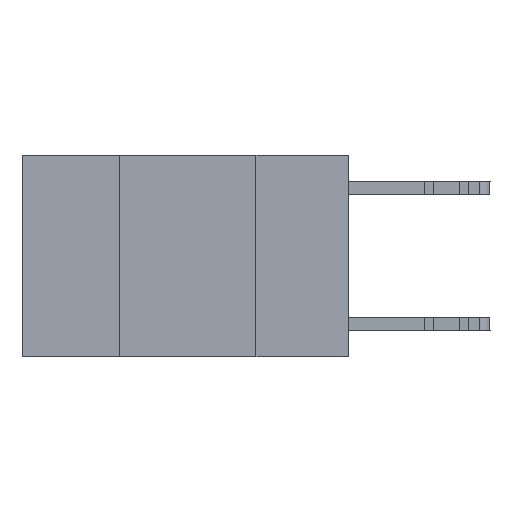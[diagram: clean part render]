
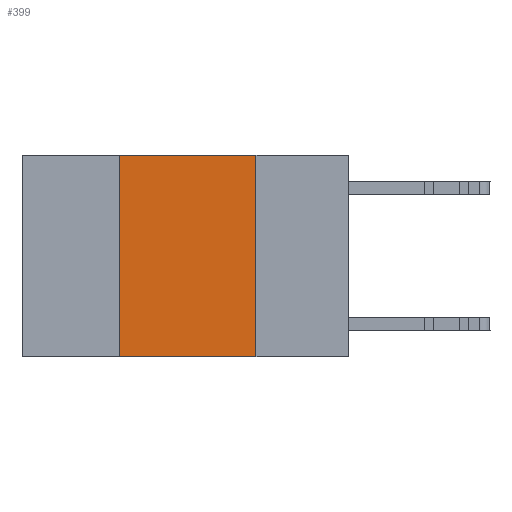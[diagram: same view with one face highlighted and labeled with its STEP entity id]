
A CAD part, left-side view. The second image highlights one B-rep face of the part: STEP entity #399.
In plain terms, the highlighted planar face has unit normal (-1, 0, 0).
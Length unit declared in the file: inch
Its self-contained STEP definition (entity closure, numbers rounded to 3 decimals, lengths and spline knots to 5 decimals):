
#399 = ADVANCED_FACE ( 'NONE', ( #556 ), #14731, .F. ) ;
#556 = FACE_OUTER_BOUND ( 'NONE', #13640, .T. ) ;
#1624 = VERTEX_POINT ( 'NONE', #8422 ) ;
#3134 = CARTESIAN_POINT ( 'NONE',  ( 0., 0.17, 0. ) ) ;
#4182 = DIRECTION ( 'NONE',  ( 0., -1., 0. ) ) ;
#5561 = DIRECTION ( 'NONE',  ( 0., -1., 0. ) ) ;
#5857 = VERTEX_POINT ( 'NONE', #28894 ) ;
#7335 = VERTEX_POINT ( 'NONE', #27470 ) ;
#8422 = CARTESIAN_POINT ( 'NONE',  ( 0., 0.42, 0. ) ) ;
#8633 = VECTOR ( 'NONE', #29550, 39.37008 ) ;
#8825 = VECTOR ( 'NONE', #4182, 39.37008 ) ;
#12946 = LINE ( 'NONE', #3134, #18181 ) ;
#13363 = CARTESIAN_POINT ( 'NONE',  ( 0., 0.6, -0.37 ) ) ;
#13640 = EDGE_LOOP ( 'NONE', ( #14396, #13932, #24331, #19366 ) ) ;
#13932 = ORIENTED_EDGE ( 'NONE', *, *, #27492, .F. ) ;
#14396 = ORIENTED_EDGE ( 'NONE', *, *, #28361, .F. ) ;
#14731 = PLANE ( 'NONE',  #17290 ) ;
#17290 = AXIS2_PLACEMENT_3D ( 'NONE', #24223, #24387, #26725 ) ;
#18181 = VECTOR ( 'NONE', #26953, 39.37008 ) ;
#19366 = ORIENTED_EDGE ( 'NONE', *, *, #30375, .T. ) ;
#20601 = VECTOR ( 'NONE', #5561, 39.37008 ) ;
#23722 = EDGE_CURVE ( 'NONE', #5857, #1624, #29701, .T. ) ;
#24223 = CARTESIAN_POINT ( 'NONE',  ( 0., 0.6, 0. ) ) ;
#24331 = ORIENTED_EDGE ( 'NONE', *, *, #23722, .F. ) ;
#24387 = DIRECTION ( 'NONE',  ( 1., 0., 0. ) ) ;
#25127 = VERTEX_POINT ( 'NONE', #27671 ) ;
#26725 = DIRECTION ( 'NONE',  ( 0., 0., -1. ) ) ;
#26953 = DIRECTION ( 'NONE',  ( 0., 0., -1. ) ) ;
#27470 = CARTESIAN_POINT ( 'NONE',  ( 0., 0.17, 0. ) ) ;
#27492 = EDGE_CURVE ( 'NONE', #1624, #7335, #29383, .T. ) ;
#27671 = CARTESIAN_POINT ( 'NONE',  ( 0., 0.17, -0.37 ) ) ;
#27777 = CARTESIAN_POINT ( 'NONE',  ( 0., 0.42, 0. ) ) ;
#28361 = EDGE_CURVE ( 'NONE', #7335, #25127, #12946, .T. ) ;
#28894 = CARTESIAN_POINT ( 'NONE',  ( 0., 0.42, -0.37 ) ) ;
#29383 = LINE ( 'NONE', #29689, #20601 ) ;
#29550 = DIRECTION ( 'NONE',  ( 0., 0., 1. ) ) ;
#29689 = CARTESIAN_POINT ( 'NONE',  ( 0., 0.6, 0. ) ) ;
#29701 = LINE ( 'NONE', #27777, #8633 ) ;
#30341 = LINE ( 'NONE', #13363, #8825 ) ;
#30375 = EDGE_CURVE ( 'NONE', #5857, #25127, #30341, .T. ) ;
